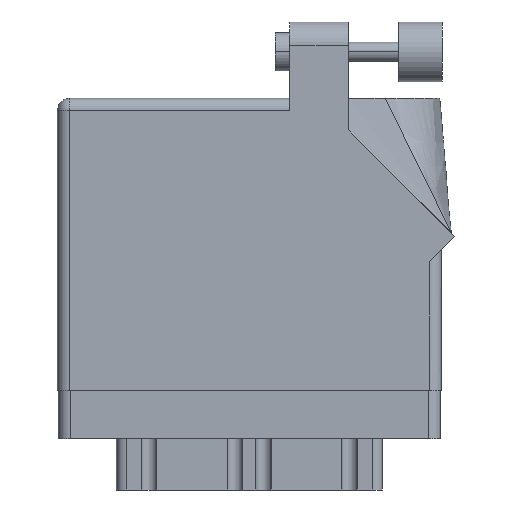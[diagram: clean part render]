
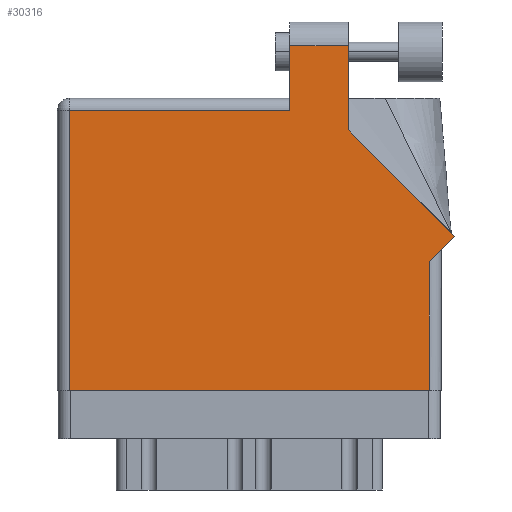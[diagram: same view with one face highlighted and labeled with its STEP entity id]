
A CAD part, front view. The second image highlights one B-rep face of the part: STEP entity #30316.
In plain terms, the highlighted face is planar.
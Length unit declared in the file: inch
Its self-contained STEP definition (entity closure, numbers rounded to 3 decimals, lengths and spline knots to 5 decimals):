
#137 = CARTESIAN_POINT ( 'NONE',  ( 2.01, 0.737, 0. ) ) ;
#735 = DIRECTION ( 'NONE',  ( 0., -1., 0. ) ) ;
#1057 = ORIENTED_EDGE ( 'NONE', *, *, #14263, .T. ) ;
#1399 = VERTEX_POINT ( 'NONE', #28278 ) ;
#2211 = DIRECTION ( 'NONE',  ( -1., 0., 0. ) ) ;
#3450 = CARTESIAN_POINT ( 'NONE',  ( 0.062, 1.468, 0. ) ) ;
#4120 = EDGE_CURVE ( 'NONE', #23647, #16486, #34311, .T. ) ;
#4313 = ORIENTED_EDGE ( 'NONE', *, *, #6048, .T. ) ;
#5619 = CARTESIAN_POINT ( 'NONE',  ( 0., 0., 0. ) ) ;
#5882 = CARTESIAN_POINT ( 'NONE',  ( 1.217, 1.805, 0. ) ) ;
#6048 = EDGE_CURVE ( 'NONE', #27218, #1399, #33532, .T. ) ;
#6577 = ORIENTED_EDGE ( 'NONE', *, *, #28907, .T. ) ;
#8420 = LINE ( 'NONE', #5619, #34620 ) ;
#8974 = VECTOR ( 'NONE', #22591, 39.37008 ) ;
#9494 = VECTOR ( 'NONE', #30909, 39.37008 ) ;
#9821 = CARTESIAN_POINT ( 'NONE',  ( 1.217, 1.468, 0. ) ) ;
#10022 = VECTOR ( 'NONE', #11503, 39.37008 ) ;
#10277 = EDGE_CURVE ( 'NONE', #16486, #10575, #21454, .T. ) ;
#10575 = VERTEX_POINT ( 'NONE', #9821 ) ;
#10762 = CARTESIAN_POINT ( 'NONE',  ( 2.08071, 0.80771, 0. ) ) ;
#11157 = ORIENTED_EDGE ( 'NONE', *, *, #31259, .T. ) ;
#11449 = LINE ( 'NONE', #10762, #25842 ) ;
#11503 = DIRECTION ( 'NONE',  ( 0., 1., 0. ) ) ;
#12259 = VERTEX_POINT ( 'NONE', #12868 ) ;
#12411 = CARTESIAN_POINT ( 'NONE',  ( 0., 1.468, 0. ) ) ;
#12796 = AXIS2_PLACEMENT_3D ( 'NONE', #19158, #23889, #32130 ) ;
#12813 = ORIENTED_EDGE ( 'NONE', *, *, #21271, .T. ) ;
#12868 = CARTESIAN_POINT ( 'NONE',  ( 0.062, 0., 0. ) ) ;
#12948 = DIRECTION ( 'NONE',  ( 0.707, 0.707, 0. ) ) ;
#13184 = FACE_OUTER_BOUND ( 'NONE', #13301, .T. ) ;
#13301 = EDGE_LOOP ( 'NONE', ( #11157, #14744, #24725, #29296, #1057, #6577, #4313, #22058, #12813 ) ) ;
#13610 = CARTESIAN_POINT ( 'NONE',  ( 1.217, 1.805, 0. ) ) ;
#14165 = CARTESIAN_POINT ( 'NONE',  ( 1.524, 1.805, 0. ) ) ;
#14263 = EDGE_CURVE ( 'NONE', #32227, #12259, #17192, .T. ) ;
#14744 = ORIENTED_EDGE ( 'NONE', *, *, #4120, .T. ) ;
#16486 = VERTEX_POINT ( 'NONE', #5882 ) ;
#17192 = LINE ( 'NONE', #27888, #25624 ) ;
#19158 = CARTESIAN_POINT ( 'NONE',  ( 0., 1.53, 0. ) ) ;
#19200 = EDGE_CURVE ( 'NONE', #10575, #32227, #23111, .T. ) ;
#20238 = CARTESIAN_POINT ( 'NONE',  ( 1.948, 0.737, 0. ) ) ;
#21271 = EDGE_CURVE ( 'NONE', #28471, #33304, #11449, .T. ) ;
#21454 = LINE ( 'NONE', #27375, #29509 ) ;
#21644 = DIRECTION ( 'NONE',  ( -0.707, 0.707, 0. ) ) ;
#21907 = EDGE_CURVE ( 'NONE', #1399, #28471, #28382, .T. ) ;
#21956 = VECTOR ( 'NONE', #12948, 39.37008 ) ;
#22058 = ORIENTED_EDGE ( 'NONE', *, *, #21907, .T. ) ;
#22490 = CARTESIAN_POINT ( 'NONE',  ( 1.524, 1.36442, 0. ) ) ;
#22591 = DIRECTION ( 'NONE',  ( -1., 0., 0. ) ) ;
#23111 = LINE ( 'NONE', #12411, #8974 ) ;
#23647 = VERTEX_POINT ( 'NONE', #14165 ) ;
#23889 = DIRECTION ( 'NONE',  ( 0., 0., -1. ) ) ;
#24567 = DIRECTION ( 'NONE',  ( 0., -1., 0. ) ) ;
#24725 = ORIENTED_EDGE ( 'NONE', *, *, #10277, .T. ) ;
#25380 = CARTESIAN_POINT ( 'NONE',  ( 1.524, 1.36442, 0. ) ) ;
#25624 = VECTOR ( 'NONE', #24567, 39.37008 ) ;
#25842 = VECTOR ( 'NONE', #21644, 39.37008 ) ;
#26032 = CARTESIAN_POINT ( 'NONE',  ( 1.948, 0., 0. ) ) ;
#26041 = CARTESIAN_POINT ( 'NONE',  ( 2.08071, 0.80771, 0. ) ) ;
#26682 = PLANE ( 'NONE',  #12796 ) ;
#27218 = VERTEX_POINT ( 'NONE', #26032 ) ;
#27375 = CARTESIAN_POINT ( 'NONE',  ( 1.217, 1.53, 0. ) ) ;
#27888 = CARTESIAN_POINT ( 'NONE',  ( 0.062, 0., 0. ) ) ;
#28278 = CARTESIAN_POINT ( 'NONE',  ( 1.948, 0.675, 0. ) ) ;
#28382 = LINE ( 'NONE', #137, #21956 ) ;
#28471 = VERTEX_POINT ( 'NONE', #26041 ) ;
#28907 = EDGE_CURVE ( 'NONE', #12259, #27218, #8420, .T. ) ;
#29153 = DIRECTION ( 'NONE',  ( 1., 0., 0. ) ) ;
#29296 = ORIENTED_EDGE ( 'NONE', *, *, #19200, .T. ) ;
#29509 = VECTOR ( 'NONE', #735, 39.37008 ) ;
#30316 = ADVANCED_FACE ( 'NONE', ( #13184 ), #26682, .F. ) ;
#30909 = DIRECTION ( 'NONE',  ( 0., 1., 0. ) ) ;
#31259 = EDGE_CURVE ( 'NONE', #33304, #23647, #33426, .T. ) ;
#31906 = VECTOR ( 'NONE', #2211, 39.37008 ) ;
#32130 = DIRECTION ( 'NONE',  ( -1., 0., 0. ) ) ;
#32227 = VERTEX_POINT ( 'NONE', #3450 ) ;
#33304 = VERTEX_POINT ( 'NONE', #22490 ) ;
#33426 = LINE ( 'NONE', #25380, #10022 ) ;
#33532 = LINE ( 'NONE', #20238, #9494 ) ;
#34311 = LINE ( 'NONE', #13610, #31906 ) ;
#34620 = VECTOR ( 'NONE', #29153, 39.37008 ) ;
